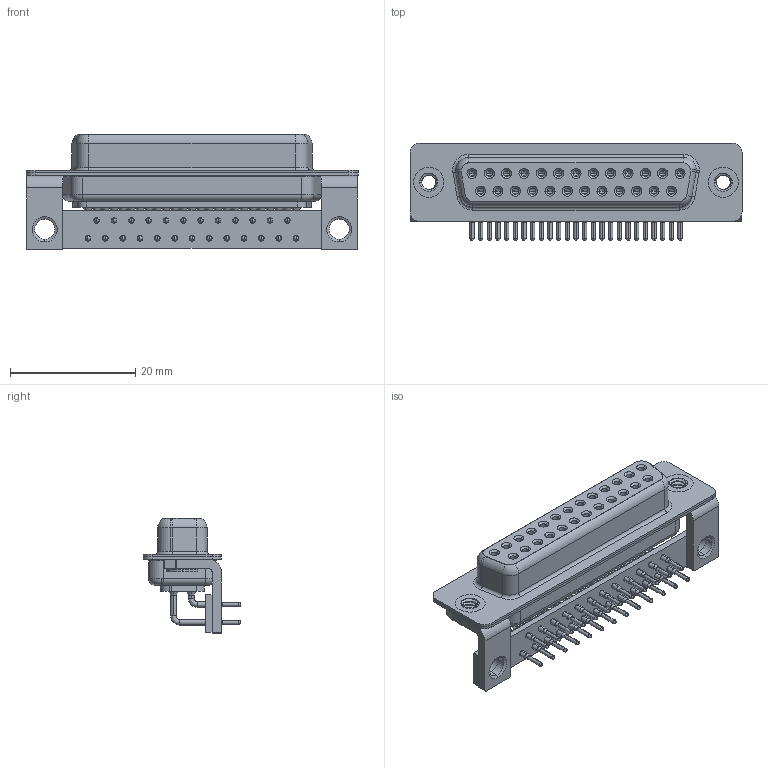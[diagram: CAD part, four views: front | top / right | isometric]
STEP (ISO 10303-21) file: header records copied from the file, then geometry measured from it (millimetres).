
FILE_DESCRIPTION (( 'STEP AP203' ), '1' );
FILE_NAME ('622-M25-660-GN4.STEP', '2018-09-24T22:12:15', ( '' ), ( '' ), 'SwSTEP 2.0', 'SolidWorks 2016', '' );
FILE_SCHEMA (( 'CONFIG_CONTROL_DESIGN' ));
Length unit declared in the file: millimetre
Products named in the file (9): 622-M25-660-GN4; 622M Housing_25 Contacts; 622M Shell Front_25 Contacts; 622M Shell Rear_25 Contacts; 622M Contact Row 1; 622M Contact Row 2; 622M 4-40 Threaded Rivet_Stabilizer; 622M Stabilizer Bracket; 622M Stabilizer Board_25 Contacts
Assembly tree (33 placements, depth 2):
  622-M25-660-GN4
    622M Housing_25 Contacts
    622M Shell Front_25 Contacts
    622M Shell Rear_25 Contacts
    622M Contact Row 1  x13
    622M Contact Row 2  x12
    622M 4-40 Threaded Rivet_Stabilizer  x2
    622M Stabilizer Bracket  x2
    622M Stabilizer Board_25 Contacts
Bounding box: 53.05 x 15.6 x 18.5 mm (x, y, z)
Volume: 4362.1 mm3; surface area: 10799.3 mm2
Topology: 33 solids, 33 shells, 1704 faces, 4342 edges, 2740 vertices
Faces by surface type: cylinder 784, plane 468, cone 283, bspline 106, torus 63
Entity records: 24978 total; most frequent: CARTESIAN_POINT 5411, DIRECTION 4131, ORIENTED_EDGE 3476, EDGE_CURVE 1738, AXIS2_PLACEMENT_3D 1726, VERTEX_POINT 1111, CIRCLE 970, EDGE_LOOP 941
